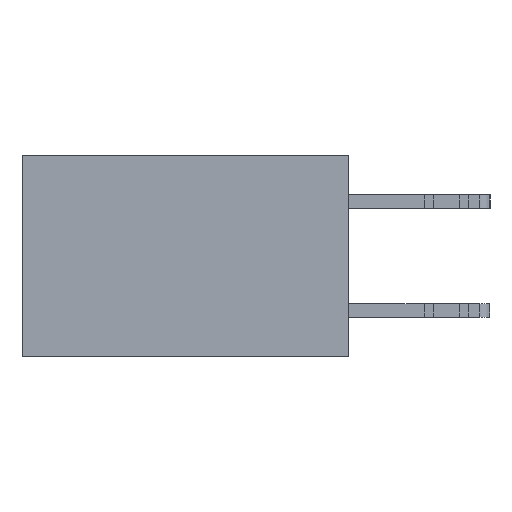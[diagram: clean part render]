
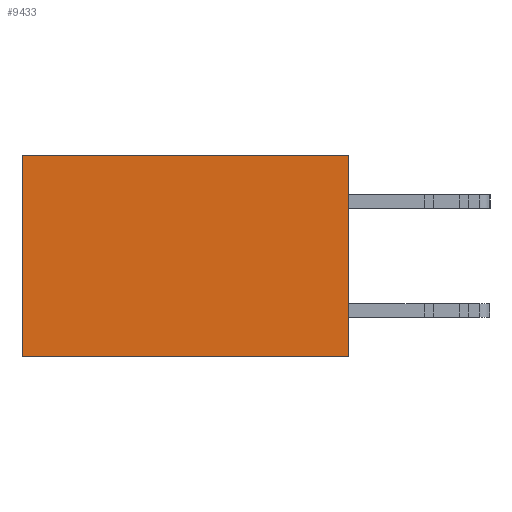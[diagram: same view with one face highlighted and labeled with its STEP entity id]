
A CAD part, left-side view. The second image highlights one B-rep face of the part: STEP entity #9433.
In plain terms, the highlighted planar face has unit normal (-1, 0, 0).
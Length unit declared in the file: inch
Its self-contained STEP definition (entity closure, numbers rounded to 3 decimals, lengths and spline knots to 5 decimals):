
#269 = AXIS2_PLACEMENT_3D ( 'NONE', #6515, #3000, #18818 ) ;
#855 = EDGE_CURVE ( 'NONE', #18263, #2951, #2629, .T. ) ;
#2629 = LINE ( 'NONE', #7047, #16397 ) ;
#2758 = DIRECTION ( 'NONE',  ( 0., 1., 0. ) ) ;
#2951 = VERTEX_POINT ( 'NONE', #3146 ) ;
#3000 = DIRECTION ( 'NONE',  ( 1., 0., 0. ) ) ;
#3146 = CARTESIAN_POINT ( 'NONE',  ( 0.2615, 0., -0.37 ) ) ;
#4400 = LINE ( 'NONE', #8157, #17990 ) ;
#5376 = DIRECTION ( 'NONE',  ( 0., 1., 0. ) ) ;
#5417 = ORIENTED_EDGE ( 'NONE', *, *, #6158, .T. ) ;
#6158 = EDGE_CURVE ( 'NONE', #18263, #12098, #9001, .T. ) ;
#6515 = CARTESIAN_POINT ( 'NONE',  ( 0.2615, 0., -0.37 ) ) ;
#7047 = CARTESIAN_POINT ( 'NONE',  ( 0.2615, 0., -0.37 ) ) ;
#8157 = CARTESIAN_POINT ( 'NONE',  ( 0.2615, 0.6, -0.37 ) ) ;
#8434 = FACE_OUTER_BOUND ( 'NONE', #20788, .T. ) ;
#9001 = LINE ( 'NONE', #24688, #22293 ) ;
#9433 = ADVANCED_FACE ( 'NONE', ( #8434 ), #24280, .F. ) ;
#9578 = ORIENTED_EDGE ( 'NONE', *, *, #25211, .F. ) ;
#10815 = DIRECTION ( 'NONE',  ( 0., 0., -1. ) ) ;
#12028 = CARTESIAN_POINT ( 'NONE',  ( 0.2615, 0.6, -0.37 ) ) ;
#12098 = VERTEX_POINT ( 'NONE', #15909 ) ;
#13905 = CARTESIAN_POINT ( 'NONE',  ( 0.2615, 0., 0. ) ) ;
#14201 = VERTEX_POINT ( 'NONE', #12028 ) ;
#14665 = LINE ( 'NONE', #17119, #22562 ) ;
#15909 = CARTESIAN_POINT ( 'NONE',  ( 0.2615, 0.6, 0. ) ) ;
#16397 = VECTOR ( 'NONE', #10815, 39.37008 ) ;
#17119 = CARTESIAN_POINT ( 'NONE',  ( 0.2615, 0., -0.37 ) ) ;
#17981 = ORIENTED_EDGE ( 'NONE', *, *, #855, .F. ) ;
#17990 = VECTOR ( 'NONE', #20082, 39.37008 ) ;
#18263 = VERTEX_POINT ( 'NONE', #13905 ) ;
#18818 = DIRECTION ( 'NONE',  ( 0., 0., -1. ) ) ;
#19177 = ORIENTED_EDGE ( 'NONE', *, *, #20444, .T. ) ;
#20082 = DIRECTION ( 'NONE',  ( 0., 0., -1. ) ) ;
#20444 = EDGE_CURVE ( 'NONE', #12098, #14201, #4400, .T. ) ;
#20788 = EDGE_LOOP ( 'NONE', ( #19177, #9578, #17981, #5417 ) ) ;
#22293 = VECTOR ( 'NONE', #5376, 39.37008 ) ;
#22562 = VECTOR ( 'NONE', #2758, 39.37008 ) ;
#24280 = PLANE ( 'NONE',  #269 ) ;
#24688 = CARTESIAN_POINT ( 'NONE',  ( 0.2615, 0., 0. ) ) ;
#25211 = EDGE_CURVE ( 'NONE', #2951, #14201, #14665, .T. ) ;
